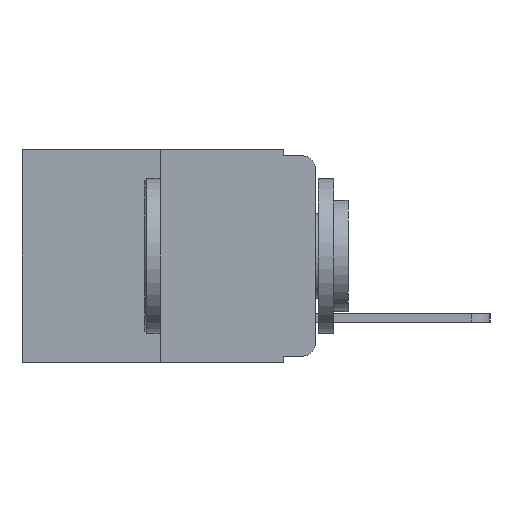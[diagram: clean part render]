
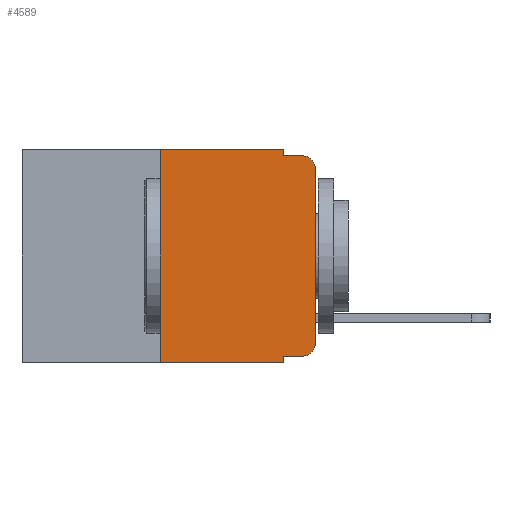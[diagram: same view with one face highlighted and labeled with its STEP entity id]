
A CAD part, left-side view. The second image highlights one B-rep face of the part: STEP entity #4589.
In plain terms, the highlighted planar face has unit normal (-1, 0, 0).
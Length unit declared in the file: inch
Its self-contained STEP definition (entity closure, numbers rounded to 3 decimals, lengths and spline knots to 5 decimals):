
#276 = DIRECTION ( 'NONE',  ( 0., -1., 0. ) ) ;
#368 = ORIENTED_EDGE ( 'NONE', *, *, #7005, .F. ) ;
#638 = LINE ( 'NONE', #3158, #4064 ) ;
#756 = EDGE_CURVE ( 'NONE', #15702, #5671, #8128, .T. ) ;
#1079 = CIRCLE ( 'NONE', #12016, 0.02 ) ;
#1094 = ORIENTED_EDGE ( 'NONE', *, *, #16751, .T. ) ;
#1193 = CARTESIAN_POINT ( 'NONE',  ( 0., 0.473, 0. ) ) ;
#1571 = DIRECTION ( 'NONE',  ( 0., -1., 0. ) ) ;
#1848 = CARTESIAN_POINT ( 'NONE',  ( 0., 0.051, -0.333 ) ) ;
#2458 = ORIENTED_EDGE ( 'NONE', *, *, #10705, .F. ) ;
#2650 = VECTOR ( 'NONE', #1571, 39.37008 ) ;
#2683 = ORIENTED_EDGE ( 'NONE', *, *, #15578, .F. ) ;
#3158 = CARTESIAN_POINT ( 'NONE',  ( 0., 0.473, 0. ) ) ;
#3225 = PLANE ( 'NONE',  #12705 ) ;
#3318 = VERTEX_POINT ( 'NONE', #15072 ) ;
#3801 = ORIENTED_EDGE ( 'NONE', *, *, #13558, .T. ) ;
#3917 = VERTEX_POINT ( 'NONE', #15128 ) ;
#4064 = VECTOR ( 'NONE', #276, 39.37008 ) ;
#4339 = CARTESIAN_POINT ( 'NONE',  ( 0., 0.25, 0. ) ) ;
#4369 = DIRECTION ( 'NONE',  ( -1., 0., 0. ) ) ;
#4493 = DIRECTION ( 'NONE',  ( 0., 0., 1. ) ) ;
#4589 = ADVANCED_FACE ( 'NONE', ( #13764 ), #3225, .F. ) ;
#5059 = DIRECTION ( 'NONE',  ( 0., 0., 1. ) ) ;
#5148 = EDGE_CURVE ( 'NONE', #3318, #9354, #8090, .T. ) ;
#5213 = DIRECTION ( 'NONE',  ( -1., 0., 0. ) ) ;
#5499 = LINE ( 'NONE', #7920, #8412 ) ;
#5631 = CARTESIAN_POINT ( 'NONE',  ( 0., 0.051, 0. ) ) ;
#5671 = VERTEX_POINT ( 'NONE', #11691 ) ;
#5948 = CARTESIAN_POINT ( 'NONE',  ( 0., 0.02, -0.01 ) ) ;
#5988 = CARTESIAN_POINT ( 'NONE',  ( 0., 0.473, -0.343 ) ) ;
#6078 = VERTEX_POINT ( 'NONE', #15231 ) ;
#6146 = CARTESIAN_POINT ( 'NONE',  ( 0., 0.051, 0. ) ) ;
#6231 = LINE ( 'NONE', #5988, #17113 ) ;
#6304 = VERTEX_POINT ( 'NONE', #10095 ) ;
#6603 = CIRCLE ( 'NONE', #17386, 0.02 ) ;
#7005 = EDGE_CURVE ( 'NONE', #5671, #14401, #10302, .T. ) ;
#7920 = CARTESIAN_POINT ( 'NONE',  ( 0., 0., 0. ) ) ;
#8090 = LINE ( 'NONE', #4339, #10999 ) ;
#8128 = LINE ( 'NONE', #6146, #14368 ) ;
#8412 = VECTOR ( 'NONE', #5059, 39.37008 ) ;
#8748 = CARTESIAN_POINT ( 'NONE',  ( 0., 0.051, -0.01 ) ) ;
#9255 = EDGE_CURVE ( 'NONE', #9374, #6078, #5499, .T. ) ;
#9354 = VERTEX_POINT ( 'NONE', #13852 ) ;
#9374 = VERTEX_POINT ( 'NONE', #16661 ) ;
#9476 = VECTOR ( 'NONE', #9978, 39.37008 ) ;
#9978 = DIRECTION ( 'NONE',  ( 0., 0., -1. ) ) ;
#10095 = CARTESIAN_POINT ( 'NONE',  ( 0., 0.051, -0.343 ) ) ;
#10302 = LINE ( 'NONE', #8748, #2650 ) ;
#10444 = VECTOR ( 'NONE', #14732, 39.37008 ) ;
#10462 = EDGE_LOOP ( 'NONE', ( #17129, #3801, #368, #16925, #2683, #15414, #1094, #2458, #10555, #15638 ) ) ;
#10555 = ORIENTED_EDGE ( 'NONE', *, *, #13091, .T. ) ;
#10705 = EDGE_CURVE ( 'NONE', #3917, #6304, #13258, .T. ) ;
#10822 = VERTEX_POINT ( 'NONE', #15824 ) ;
#10999 = VECTOR ( 'NONE', #4493, 39.37008 ) ;
#11691 = CARTESIAN_POINT ( 'NONE',  ( 0., 0.051, -0.01 ) ) ;
#12016 = AXIS2_PLACEMENT_3D ( 'NONE', #13759, #5213, #15173 ) ;
#12705 = AXIS2_PLACEMENT_3D ( 'NONE', #1193, #18184, #16291 ) ;
#12928 = CARTESIAN_POINT ( 'NONE',  ( 0., 0.02, -0.03 ) ) ;
#13091 = EDGE_CURVE ( 'NONE', #3917, #10822, #14216, .T. ) ;
#13258 = LINE ( 'NONE', #5631, #9476 ) ;
#13558 = EDGE_CURVE ( 'NONE', #6078, #14401, #6603, .T. ) ;
#13759 = CARTESIAN_POINT ( 'NONE',  ( 0., 0.02, -0.313 ) ) ;
#13764 = FACE_OUTER_BOUND ( 'NONE', #10462, .T. ) ;
#13852 = CARTESIAN_POINT ( 'NONE',  ( 0., 0.25, 0. ) ) ;
#14216 = LINE ( 'NONE', #1848, #10444 ) ;
#14355 = DIRECTION ( 'NONE',  ( 0., 0., -1. ) ) ;
#14368 = VECTOR ( 'NONE', #17849, 39.37008 ) ;
#14401 = VERTEX_POINT ( 'NONE', #5948 ) ;
#14732 = DIRECTION ( 'NONE',  ( 0., -1., 0. ) ) ;
#14892 = CARTESIAN_POINT ( 'NONE',  ( 0., 0.051, 0. ) ) ;
#15072 = CARTESIAN_POINT ( 'NONE',  ( 0., 0.25, -0.343 ) ) ;
#15128 = CARTESIAN_POINT ( 'NONE',  ( 0., 0.051, -0.333 ) ) ;
#15173 = DIRECTION ( 'NONE',  ( 0., 0., -1. ) ) ;
#15231 = CARTESIAN_POINT ( 'NONE',  ( 0., 0., -0.03 ) ) ;
#15414 = ORIENTED_EDGE ( 'NONE', *, *, #5148, .F. ) ;
#15578 = EDGE_CURVE ( 'NONE', #9354, #15702, #638, .T. ) ;
#15638 = ORIENTED_EDGE ( 'NONE', *, *, #16392, .T. ) ;
#15702 = VERTEX_POINT ( 'NONE', #14892 ) ;
#15824 = CARTESIAN_POINT ( 'NONE',  ( 0., 0.02, -0.333 ) ) ;
#15949 = DIRECTION ( 'NONE',  ( 0., -1., 0. ) ) ;
#16291 = DIRECTION ( 'NONE',  ( 0., 0., -1. ) ) ;
#16392 = EDGE_CURVE ( 'NONE', #10822, #9374, #1079, .T. ) ;
#16661 = CARTESIAN_POINT ( 'NONE',  ( 0., 0., -0.313 ) ) ;
#16751 = EDGE_CURVE ( 'NONE', #3318, #6304, #6231, .T. ) ;
#16925 = ORIENTED_EDGE ( 'NONE', *, *, #756, .F. ) ;
#17113 = VECTOR ( 'NONE', #15949, 39.37008 ) ;
#17129 = ORIENTED_EDGE ( 'NONE', *, *, #9255, .T. ) ;
#17386 = AXIS2_PLACEMENT_3D ( 'NONE', #12928, #4369, #14355 ) ;
#17849 = DIRECTION ( 'NONE',  ( 0., 0., -1. ) ) ;
#18184 = DIRECTION ( 'NONE',  ( 1., 0., 0. ) ) ;
